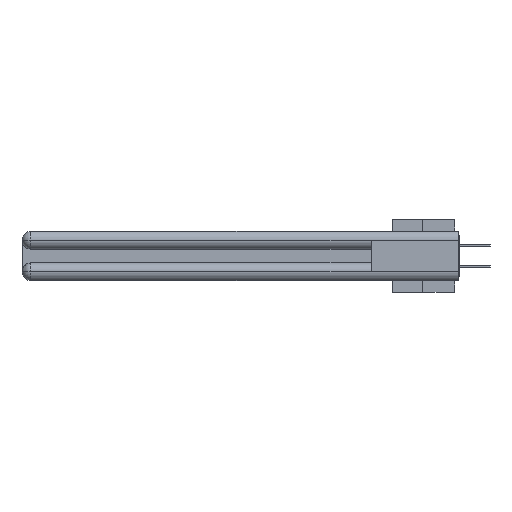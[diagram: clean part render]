
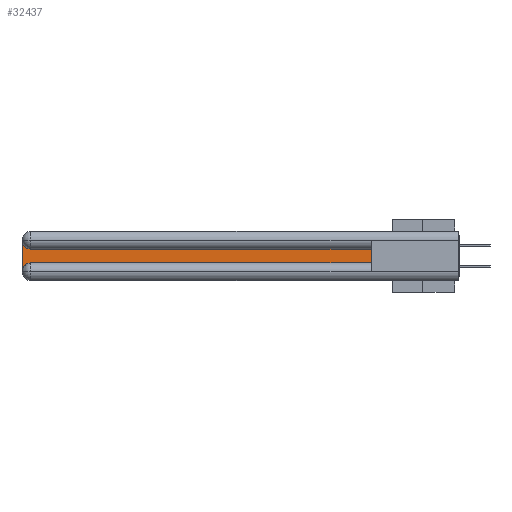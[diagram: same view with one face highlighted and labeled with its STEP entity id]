
A CAD part, left-side view. The second image highlights one B-rep face of the part: STEP entity #32437.
In plain terms, the highlighted planar face has unit normal (-1, 0, 0).
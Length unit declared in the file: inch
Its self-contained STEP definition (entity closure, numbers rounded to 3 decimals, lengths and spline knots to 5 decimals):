
#2820 = CARTESIAN_POINT ( 'NONE',  ( 0.075, 3., -0.1225 ) ) ;
#2878 = ORIENTED_EDGE ( 'NONE', *, *, #15802, .T. ) ;
#3668 = ORIENTED_EDGE ( 'NONE', *, *, #20253, .T. ) ;
#5440 = CARTESIAN_POINT ( 'NONE',  ( 0.075, 0.6, -0.1225 ) ) ;
#6236 = FACE_OUTER_BOUND ( 'NONE', #13704, .T. ) ;
#7154 = EDGE_CURVE ( 'NONE', #14889, #22724, #25762, .T. ) ;
#8339 = CARTESIAN_POINT ( 'NONE',  ( 0.075, 2.94, -0.0625 ) ) ;
#10080 = CARTESIAN_POINT ( 'NONE',  ( 0.075, 2.94, -0.2175 ) ) ;
#10194 = AXIS2_PLACEMENT_3D ( 'NONE', #2820, #38665, #20429 ) ;
#10386 = CARTESIAN_POINT ( 'NONE',  ( 0.075, 0.6, -0.2175 ) ) ;
#10705 = CARTESIAN_POINT ( 'NONE',  ( 0.075, 2.94, -0.1225 ) ) ;
#11934 = DIRECTION ( 'NONE',  ( 0., 0., 1. ) ) ;
#13704 = EDGE_LOOP ( 'NONE', ( #2878, #31801, #35770, #3668, #14337, #26723 ) ) ;
#14337 = ORIENTED_EDGE ( 'NONE', *, *, #33449, .T. ) ;
#14889 = VERTEX_POINT ( 'NONE', #10386 ) ;
#15700 = LINE ( 'NONE', #16115, #35675 ) ;
#15802 = EDGE_CURVE ( 'NONE', #22724, #33615, #26840, .T. ) ;
#15874 = CARTESIAN_POINT ( 'NONE',  ( 0.075, 0.6, -0.2175 ) ) ;
#16115 = CARTESIAN_POINT ( 'NONE',  ( 0.075, 3., -0.2175 ) ) ;
#16205 = DIRECTION ( 'NONE',  ( 1., 0., 0. ) ) ;
#16456 = VERTEX_POINT ( 'NONE', #20781 ) ;
#17380 = PLANE ( 'NONE',  #10194 ) ;
#18764 = AXIS2_PLACEMENT_3D ( 'NONE', #21916, #16205, #28334 ) ;
#20253 = EDGE_CURVE ( 'NONE', #35138, #33302, #25598, .T. ) ;
#20429 = DIRECTION ( 'NONE',  ( 0., 0., -1. ) ) ;
#20781 = CARTESIAN_POINT ( 'NONE',  ( 0.075, 3., -0.0625 ) ) ;
#21916 = CARTESIAN_POINT ( 'NONE',  ( 0.075, 2.94, -0.2775 ) ) ;
#22229 = AXIS2_PLACEMENT_3D ( 'NONE', #8339, #23193, #27060 ) ;
#22381 = DIRECTION ( 'NONE',  ( 0., -1., 0. ) ) ;
#22391 = DIRECTION ( 'NONE',  ( 0., 1., 0. ) ) ;
#22724 = VERTEX_POINT ( 'NONE', #5440 ) ;
#23193 = DIRECTION ( 'NONE',  ( 1., 0., 0. ) ) ;
#23806 = VECTOR ( 'NONE', #11934, 39.37008 ) ;
#24633 = LINE ( 'NONE', #15874, #36032 ) ;
#25581 = EDGE_CURVE ( 'NONE', #33615, #16456, #36297, .T. ) ;
#25598 = CIRCLE ( 'NONE', #18764, 0.06 ) ;
#25762 = LINE ( 'NONE', #36632, #23806 ) ;
#25925 = CARTESIAN_POINT ( 'NONE',  ( 0.075, 3., -0.2775 ) ) ;
#26723 = ORIENTED_EDGE ( 'NONE', *, *, #7154, .T. ) ;
#26840 = LINE ( 'NONE', #34095, #35398 ) ;
#27060 = DIRECTION ( 'NONE',  ( 0., 0., -1. ) ) ;
#27348 = EDGE_CURVE ( 'NONE', #16456, #35138, #15700, .T. ) ;
#28334 = DIRECTION ( 'NONE',  ( 0., 0., -1. ) ) ;
#31801 = ORIENTED_EDGE ( 'NONE', *, *, #25581, .T. ) ;
#32437 = ADVANCED_FACE ( 'NONE', ( #6236 ), #17380, .F. ) ;
#33302 = VERTEX_POINT ( 'NONE', #10080 ) ;
#33449 = EDGE_CURVE ( 'NONE', #33302, #14889, #24633, .T. ) ;
#33615 = VERTEX_POINT ( 'NONE', #10705 ) ;
#34095 = CARTESIAN_POINT ( 'NONE',  ( 0.075, 0.6, -0.1225 ) ) ;
#35138 = VERTEX_POINT ( 'NONE', #25925 ) ;
#35398 = VECTOR ( 'NONE', #22391, 39.37008 ) ;
#35675 = VECTOR ( 'NONE', #36990, 39.37008 ) ;
#35770 = ORIENTED_EDGE ( 'NONE', *, *, #27348, .T. ) ;
#36032 = VECTOR ( 'NONE', #22381, 39.37008 ) ;
#36297 = CIRCLE ( 'NONE', #22229, 0.06 ) ;
#36632 = CARTESIAN_POINT ( 'NONE',  ( 0.075, 0.6, -0.2175 ) ) ;
#36990 = DIRECTION ( 'NONE',  ( 0., 0., -1. ) ) ;
#38665 = DIRECTION ( 'NONE',  ( 1., 0., 0. ) ) ;
